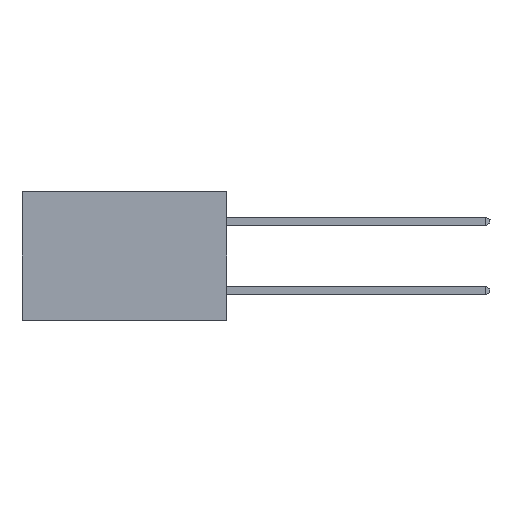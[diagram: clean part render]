
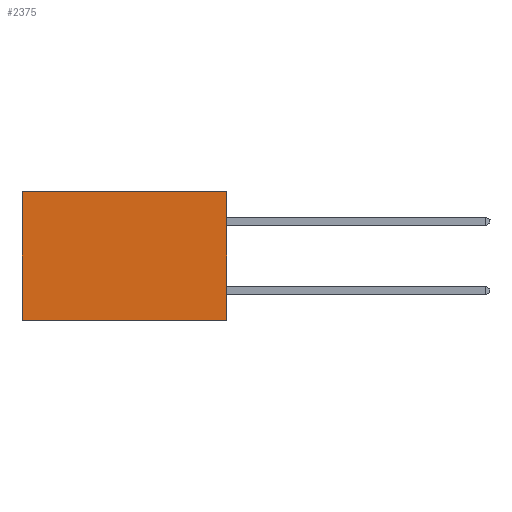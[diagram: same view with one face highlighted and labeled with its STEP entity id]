
A CAD part, left-side view. The second image highlights one B-rep face of the part: STEP entity #2375.
In plain terms, the highlighted planar face has unit normal (-1, 0, 0).
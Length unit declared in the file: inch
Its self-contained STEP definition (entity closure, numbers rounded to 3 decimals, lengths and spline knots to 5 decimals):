
#258 = LINE ( 'NONE', #3604, #6993 ) ;
#484 = CARTESIAN_POINT ( 'NONE',  ( 0.277, 0.59, 0. ) ) ;
#816 = DIRECTION ( 'NONE',  ( 0., 1., 0. ) ) ;
#884 = VERTEX_POINT ( 'NONE', #484 ) ;
#915 = VERTEX_POINT ( 'NONE', #2213 ) ;
#1788 = VECTOR ( 'NONE', #816, 39.37008 ) ;
#2213 = CARTESIAN_POINT ( 'NONE',  ( 0.277, 0., 0. ) ) ;
#2375 = ADVANCED_FACE ( 'NONE', ( #7099 ), #8764, .F. ) ;
#2723 = ORIENTED_EDGE ( 'NONE', *, *, #8103, .F. ) ;
#3002 = EDGE_CURVE ( 'NONE', #3873, #5170, #10695, .T. ) ;
#3246 = VECTOR ( 'NONE', #7770, 39.37008 ) ;
#3267 = CARTESIAN_POINT ( 'NONE',  ( 0.277, 0., -0.37 ) ) ;
#3409 = EDGE_CURVE ( 'NONE', #884, #5170, #5928, .T. ) ;
#3532 = VECTOR ( 'NONE', #10187, 39.37008 ) ;
#3604 = CARTESIAN_POINT ( 'NONE',  ( 0.277, 0., -0.37 ) ) ;
#3873 = VERTEX_POINT ( 'NONE', #6692 ) ;
#3877 = AXIS2_PLACEMENT_3D ( 'NONE', #11503, #8804, #8370 ) ;
#4555 = LINE ( 'NONE', #10720, #1788 ) ;
#4596 = ORIENTED_EDGE ( 'NONE', *, *, #3002, .F. ) ;
#5170 = VERTEX_POINT ( 'NONE', #6428 ) ;
#5928 = LINE ( 'NONE', #10878, #3532 ) ;
#6330 = DIRECTION ( 'NONE',  ( 0., 0., -1. ) ) ;
#6428 = CARTESIAN_POINT ( 'NONE',  ( 0.277, 0.59, -0.37 ) ) ;
#6692 = CARTESIAN_POINT ( 'NONE',  ( 0.277, 0., -0.37 ) ) ;
#6993 = VECTOR ( 'NONE', #6330, 39.37008 ) ;
#7099 = FACE_OUTER_BOUND ( 'NONE', #11506, .T. ) ;
#7770 = DIRECTION ( 'NONE',  ( 0., 1., 0. ) ) ;
#8103 = EDGE_CURVE ( 'NONE', #915, #3873, #258, .T. ) ;
#8370 = DIRECTION ( 'NONE',  ( 0., 0., -1. ) ) ;
#8764 = PLANE ( 'NONE',  #3877 ) ;
#8804 = DIRECTION ( 'NONE',  ( 1., 0., 0. ) ) ;
#9100 = ORIENTED_EDGE ( 'NONE', *, *, #3409, .T. ) ;
#10187 = DIRECTION ( 'NONE',  ( 0., 0., -1. ) ) ;
#10474 = ORIENTED_EDGE ( 'NONE', *, *, #10548, .T. ) ;
#10548 = EDGE_CURVE ( 'NONE', #915, #884, #4555, .T. ) ;
#10695 = LINE ( 'NONE', #3267, #3246 ) ;
#10720 = CARTESIAN_POINT ( 'NONE',  ( 0.277, 0., 0. ) ) ;
#10878 = CARTESIAN_POINT ( 'NONE',  ( 0.277, 0.59, -0.37 ) ) ;
#11503 = CARTESIAN_POINT ( 'NONE',  ( 0.277, 0., -0.37 ) ) ;
#11506 = EDGE_LOOP ( 'NONE', ( #9100, #4596, #2723, #10474 ) ) ;
